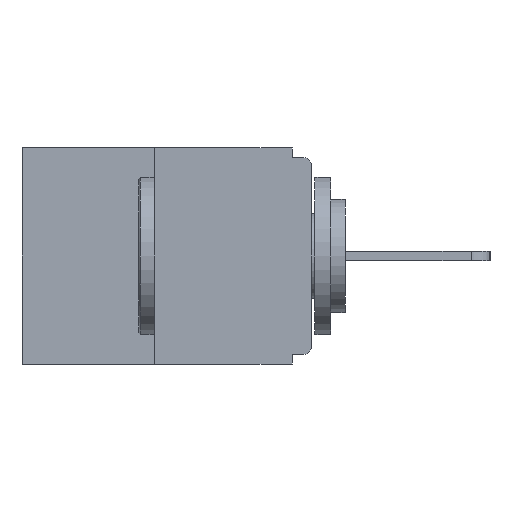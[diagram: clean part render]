
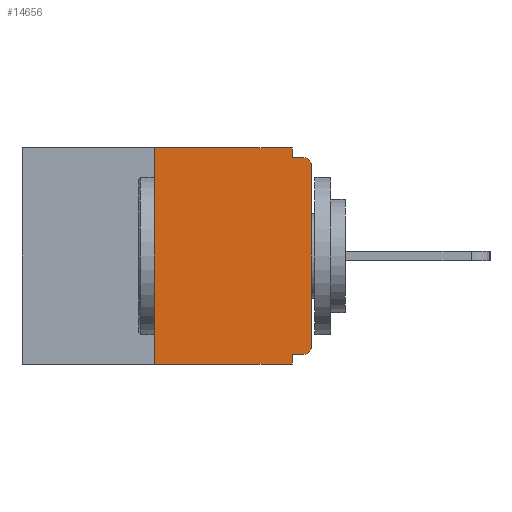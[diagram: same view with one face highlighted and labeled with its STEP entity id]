
A CAD part, left-side view. The second image highlights one B-rep face of the part: STEP entity #14656.
In plain terms, the highlighted planar face has unit normal (-1, 0, 0).
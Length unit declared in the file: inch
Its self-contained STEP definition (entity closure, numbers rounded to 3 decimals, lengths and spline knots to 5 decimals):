
#154 = EDGE_CURVE ( 'NONE', #2546, #7959, #10008, .T. ) ;
#330 = VECTOR ( 'NONE', #542, 39.37008 ) ;
#542 = DIRECTION ( 'NONE',  ( 0., 1., 0. ) ) ;
#736 = DIRECTION ( 'NONE',  ( 1., 0., 0. ) ) ;
#831 = EDGE_LOOP ( 'NONE', ( #10716, #16038, #6538, #7593, #1507, #8358, #3511, #10616, #15927, #5042 ) ) ;
#965 = LINE ( 'NONE', #14904, #15647 ) ;
#1063 = DIRECTION ( 'NONE',  ( 0., 0., 1. ) ) ;
#1291 = DIRECTION ( 'NONE',  ( -1., 0., 0. ) ) ;
#1362 = CARTESIAN_POINT ( 'NONE',  ( 0., 0.46, 0. ) ) ;
#1473 = VERTEX_POINT ( 'NONE', #15989 ) ;
#1507 = ORIENTED_EDGE ( 'NONE', *, *, #12452, .F. ) ;
#1855 = CARTESIAN_POINT ( 'NONE',  ( 0., 0., -0.328 ) ) ;
#1961 = PLANE ( 'NONE',  #15105 ) ;
#2013 = VERTEX_POINT ( 'NONE', #4405 ) ;
#2104 = CARTESIAN_POINT ( 'NONE',  ( 0., 0.015, -0.328 ) ) ;
#2192 = LINE ( 'NONE', #8497, #4071 ) ;
#2199 = VECTOR ( 'NONE', #1063, 39.37008 ) ;
#2260 = CARTESIAN_POINT ( 'NONE',  ( 0., 0., 0. ) ) ;
#2419 = EDGE_CURVE ( 'NONE', #10759, #1473, #15978, .T. ) ;
#2546 = VERTEX_POINT ( 'NONE', #2104 ) ;
#2856 = VERTEX_POINT ( 'NONE', #9539 ) ;
#2876 = AXIS2_PLACEMENT_3D ( 'NONE', #7021, #8361, #11863 ) ;
#2956 = CARTESIAN_POINT ( 'NONE',  ( 0., 0.031, 0. ) ) ;
#3263 = VECTOR ( 'NONE', #6436, 39.37008 ) ;
#3363 = DIRECTION ( 'NONE',  ( 0., -1., 0. ) ) ;
#3511 = ORIENTED_EDGE ( 'NONE', *, *, #7721, .T. ) ;
#4071 = VECTOR ( 'NONE', #13411, 39.37008 ) ;
#4405 = CARTESIAN_POINT ( 'NONE',  ( 0., 0.25, -0.343 ) ) ;
#5042 = ORIENTED_EDGE ( 'NONE', *, *, #15117, .F. ) ;
#5221 = EDGE_CURVE ( 'NONE', #5249, #1473, #9298, .T. ) ;
#5249 = VERTEX_POINT ( 'NONE', #10063 ) ;
#5399 = CARTESIAN_POINT ( 'NONE',  ( 0., 0., -0.313 ) ) ;
#5853 = VECTOR ( 'NONE', #14411, 39.37008 ) ;
#6436 = DIRECTION ( 'NONE',  ( 0., -1., 0. ) ) ;
#6538 = ORIENTED_EDGE ( 'NONE', *, *, #15061, .T. ) ;
#6783 = CARTESIAN_POINT ( 'NONE',  ( 0., 0.25, 0. ) ) ;
#7014 = LINE ( 'NONE', #14580, #5853 ) ;
#7021 = CARTESIAN_POINT ( 'NONE',  ( 0., 0.015, -0.313 ) ) ;
#7028 = DIRECTION ( 'NONE',  ( 0., 0., -1. ) ) ;
#7121 = EDGE_CURVE ( 'NONE', #8330, #2856, #7014, .T. ) ;
#7403 = DIRECTION ( 'NONE',  ( 0., 0., -1. ) ) ;
#7593 = ORIENTED_EDGE ( 'NONE', *, *, #7121, .F. ) ;
#7718 = AXIS2_PLACEMENT_3D ( 'NONE', #8930, #1291, #16314 ) ;
#7721 = EDGE_CURVE ( 'NONE', #7959, #5249, #7996, .T. ) ;
#7959 = VERTEX_POINT ( 'NONE', #5399 ) ;
#7996 = LINE ( 'NONE', #2260, #9561 ) ;
#8330 = VERTEX_POINT ( 'NONE', #15023 ) ;
#8358 = ORIENTED_EDGE ( 'NONE', *, *, #154, .T. ) ;
#8361 = DIRECTION ( 'NONE',  ( -1., 0., 0. ) ) ;
#8497 = CARTESIAN_POINT ( 'NONE',  ( 0., 0.46, -0.343 ) ) ;
#8930 = CARTESIAN_POINT ( 'NONE',  ( 0., 0.015, -0.03 ) ) ;
#9298 = CIRCLE ( 'NONE', #7718, 0.015 ) ;
#9539 = CARTESIAN_POINT ( 'NONE',  ( 0., 0.031, -0.343 ) ) ;
#9561 = VECTOR ( 'NONE', #12161, 39.37008 ) ;
#9582 = CARTESIAN_POINT ( 'NONE',  ( 0., 0.031, -0.015 ) ) ;
#9697 = LINE ( 'NONE', #14697, #2199 ) ;
#10008 = CIRCLE ( 'NONE', #2876, 0.015 ) ;
#10063 = CARTESIAN_POINT ( 'NONE',  ( 0., 0., -0.03 ) ) ;
#10144 = LINE ( 'NONE', #1362, #3263 ) ;
#10535 = VERTEX_POINT ( 'NONE', #6783 ) ;
#10616 = ORIENTED_EDGE ( 'NONE', *, *, #5221, .T. ) ;
#10716 = ORIENTED_EDGE ( 'NONE', *, *, #14892, .F. ) ;
#10759 = VERTEX_POINT ( 'NONE', #9582 ) ;
#10794 = LINE ( 'NONE', #1855, #330 ) ;
#11863 = DIRECTION ( 'NONE',  ( 0., 0., -1. ) ) ;
#11868 = CARTESIAN_POINT ( 'NONE',  ( 0., 0.46, 0. ) ) ;
#11894 = VECTOR ( 'NONE', #3363, 39.37008 ) ;
#12161 = DIRECTION ( 'NONE',  ( 0., 0., 1. ) ) ;
#12452 = EDGE_CURVE ( 'NONE', #2546, #8330, #10794, .T. ) ;
#12916 = EDGE_CURVE ( 'NONE', #2013, #10535, #9697, .T. ) ;
#13097 = FACE_OUTER_BOUND ( 'NONE', #831, .T. ) ;
#13411 = DIRECTION ( 'NONE',  ( 0., -1., 0. ) ) ;
#14411 = DIRECTION ( 'NONE',  ( 0., 0., -1. ) ) ;
#14576 = CARTESIAN_POINT ( 'NONE',  ( 0., 0., -0.015 ) ) ;
#14580 = CARTESIAN_POINT ( 'NONE',  ( 0., 0.031, -0.343 ) ) ;
#14632 = VERTEX_POINT ( 'NONE', #2956 ) ;
#14656 = ADVANCED_FACE ( 'NONE', ( #13097 ), #1961, .F. ) ;
#14697 = CARTESIAN_POINT ( 'NONE',  ( 0., 0.25, 0. ) ) ;
#14892 = EDGE_CURVE ( 'NONE', #10535, #14632, #10144, .T. ) ;
#14904 = CARTESIAN_POINT ( 'NONE',  ( 0., 0.031, 0. ) ) ;
#15023 = CARTESIAN_POINT ( 'NONE',  ( 0., 0.031, -0.328 ) ) ;
#15061 = EDGE_CURVE ( 'NONE', #2013, #2856, #2192, .T. ) ;
#15105 = AXIS2_PLACEMENT_3D ( 'NONE', #11868, #736, #7028 ) ;
#15117 = EDGE_CURVE ( 'NONE', #14632, #10759, #965, .T. ) ;
#15647 = VECTOR ( 'NONE', #7403, 39.37008 ) ;
#15927 = ORIENTED_EDGE ( 'NONE', *, *, #2419, .F. ) ;
#15978 = LINE ( 'NONE', #14576, #11894 ) ;
#15989 = CARTESIAN_POINT ( 'NONE',  ( 0., 0.015, -0.015 ) ) ;
#16038 = ORIENTED_EDGE ( 'NONE', *, *, #12916, .F. ) ;
#16314 = DIRECTION ( 'NONE',  ( 0., 0., -1. ) ) ;
